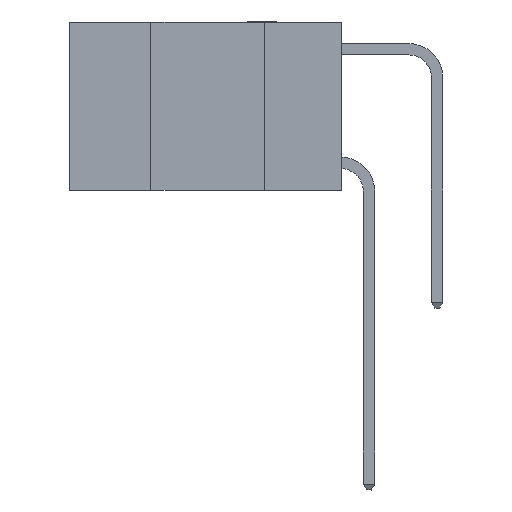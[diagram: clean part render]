
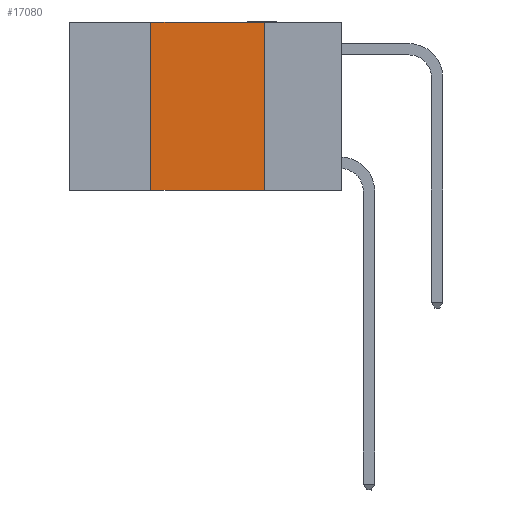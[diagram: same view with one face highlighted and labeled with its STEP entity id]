
A CAD part, left-side view. The second image highlights one B-rep face of the part: STEP entity #17080.
In plain terms, the highlighted planar face has unit normal (-1, 0, 0).
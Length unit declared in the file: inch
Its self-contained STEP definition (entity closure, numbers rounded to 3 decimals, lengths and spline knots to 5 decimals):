
#1005 = PLANE ( 'NONE',  #13965 ) ;
#2440 = EDGE_CURVE ( 'NONE', #2447, #9554, #8974, .T. ) ;
#2447 = VERTEX_POINT ( 'NONE', #17096 ) ;
#2558 = DIRECTION ( 'NONE',  ( 0., 0., 1. ) ) ;
#3354 = EDGE_CURVE ( 'NONE', #9616, #9554, #16529, .T. ) ;
#3675 = LINE ( 'NONE', #8274, #6892 ) ;
#3773 = EDGE_CURVE ( 'NONE', #2447, #9588, #6148, .T. ) ;
#3775 = DIRECTION ( 'NONE',  ( 1., 0., 0. ) ) ;
#4215 = DIRECTION ( 'NONE',  ( 0., -1., 0. ) ) ;
#4302 = CARTESIAN_POINT ( 'NONE',  ( 0., 0.17, 0. ) ) ;
#4918 = DIRECTION ( 'NONE',  ( 0., -1., 0. ) ) ;
#6067 = EDGE_LOOP ( 'NONE', ( #7770, #7865, #8185, #8238 ) ) ;
#6148 = LINE ( 'NONE', #9362, #16511 ) ;
#6419 = CARTESIAN_POINT ( 'NONE',  ( 0., 0.17, -0.37 ) ) ;
#6892 = VECTOR ( 'NONE', #4215, 39.37008 ) ;
#7770 = ORIENTED_EDGE ( 'NONE', *, *, #3354, .F. ) ;
#7865 = ORIENTED_EDGE ( 'NONE', *, *, #9110, .F. ) ;
#8185 = ORIENTED_EDGE ( 'NONE', *, *, #3773, .F. ) ;
#8238 = ORIENTED_EDGE ( 'NONE', *, *, #2440, .T. ) ;
#8274 = CARTESIAN_POINT ( 'NONE',  ( 0., 0.6, 0. ) ) ;
#8974 = LINE ( 'NONE', #10358, #12193 ) ;
#9110 = EDGE_CURVE ( 'NONE', #9588, #9616, #3675, .T. ) ;
#9362 = CARTESIAN_POINT ( 'NONE',  ( 0., 0.42, 0. ) ) ;
#9554 = VERTEX_POINT ( 'NONE', #6419 ) ;
#9588 = VERTEX_POINT ( 'NONE', #15932 ) ;
#9616 = VERTEX_POINT ( 'NONE', #13336 ) ;
#10358 = CARTESIAN_POINT ( 'NONE',  ( 0., 0.6, -0.37 ) ) ;
#11962 = CARTESIAN_POINT ( 'NONE',  ( 0., 0.6, 0. ) ) ;
#12193 = VECTOR ( 'NONE', #4918, 39.37008 ) ;
#12496 = DIRECTION ( 'NONE',  ( 0., 0., -1. ) ) ;
#13016 = VECTOR ( 'NONE', #12496, 39.37008 ) ;
#13328 = DIRECTION ( 'NONE',  ( 0., 0., -1. ) ) ;
#13336 = CARTESIAN_POINT ( 'NONE',  ( 0., 0.17, 0. ) ) ;
#13965 = AXIS2_PLACEMENT_3D ( 'NONE', #11962, #3775, #13328 ) ;
#15100 = FACE_OUTER_BOUND ( 'NONE', #6067, .T. ) ;
#15932 = CARTESIAN_POINT ( 'NONE',  ( 0., 0.42, 0. ) ) ;
#16511 = VECTOR ( 'NONE', #2558, 39.37008 ) ;
#16529 = LINE ( 'NONE', #4302, #13016 ) ;
#17080 = ADVANCED_FACE ( 'NONE', ( #15100 ), #1005, .F. ) ;
#17096 = CARTESIAN_POINT ( 'NONE',  ( 0., 0.42, -0.37 ) ) ;
